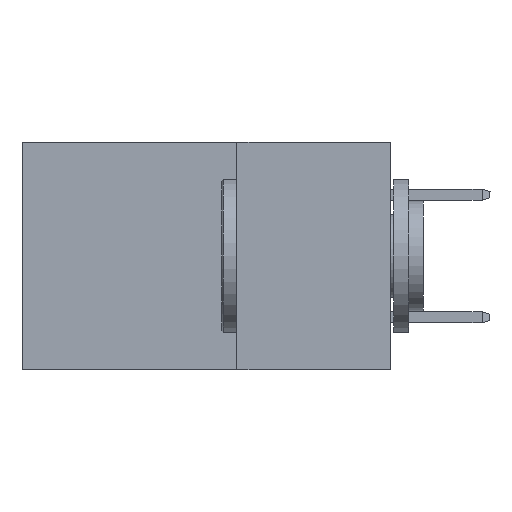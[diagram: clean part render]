
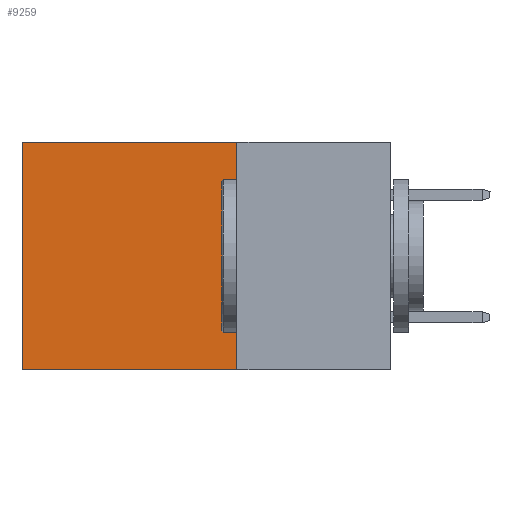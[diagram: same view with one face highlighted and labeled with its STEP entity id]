
A CAD part, left-side view. The second image highlights one B-rep face of the part: STEP entity #9259.
In plain terms, the highlighted planar face has unit normal (-1, 0, 0).
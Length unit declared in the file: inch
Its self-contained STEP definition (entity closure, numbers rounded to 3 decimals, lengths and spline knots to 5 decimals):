
#1408 = LINE ( 'NONE', #2600, #30522 ) ;
#2378 = EDGE_CURVE ( 'NONE', #23301, #19494, #18759, .T. ) ;
#2600 = CARTESIAN_POINT ( 'NONE',  ( 0.2875, 0.6, 0. ) ) ;
#3869 = EDGE_CURVE ( 'NONE', #27335, #26759, #1408, .T. ) ;
#3931 = CARTESIAN_POINT ( 'NONE',  ( 0.2875, 0.25, 0. ) ) ;
#6748 = DIRECTION ( 'NONE',  ( 0., 1., 0. ) ) ;
#7465 = DIRECTION ( 'NONE',  ( 0., 0., -1. ) ) ;
#8483 = CARTESIAN_POINT ( 'NONE',  ( 0.2875, 0.25, -0.37 ) ) ;
#8795 = LINE ( 'NONE', #33313, #10256 ) ;
#9259 = ADVANCED_FACE ( 'NONE', ( #20564 ), #22550, .F. ) ;
#10256 = VECTOR ( 'NONE', #15009, 39.37008 ) ;
#11259 = EDGE_LOOP ( 'NONE', ( #24475, #34367, #26622, #31666 ) ) ;
#12749 = EDGE_CURVE ( 'NONE', #23301, #27335, #38984, .T. ) ;
#13097 = CARTESIAN_POINT ( 'NONE',  ( 0.2875, 0.25, 0. ) ) ;
#13648 = CARTESIAN_POINT ( 'NONE',  ( 0.2875, 0.6, 0. ) ) ;
#15009 = DIRECTION ( 'NONE',  ( 0., 1., 0. ) ) ;
#15402 = AXIS2_PLACEMENT_3D ( 'NONE', #3931, #25070, #34419 ) ;
#18759 = LINE ( 'NONE', #28833, #38855 ) ;
#18828 = CARTESIAN_POINT ( 'NONE',  ( 0.2875, 0.25, 0. ) ) ;
#19494 = VERTEX_POINT ( 'NONE', #8483 ) ;
#20564 = FACE_OUTER_BOUND ( 'NONE', #11259, .T. ) ;
#22550 = PLANE ( 'NONE',  #15402 ) ;
#22758 = VECTOR ( 'NONE', #6748, 39.37008 ) ;
#23301 = VERTEX_POINT ( 'NONE', #18828 ) ;
#24475 = ORIENTED_EDGE ( 'NONE', *, *, #3869, .T. ) ;
#25070 = DIRECTION ( 'NONE',  ( 1., 0., 0. ) ) ;
#26622 = ORIENTED_EDGE ( 'NONE', *, *, #2378, .F. ) ;
#26759 = VERTEX_POINT ( 'NONE', #30993 ) ;
#27335 = VERTEX_POINT ( 'NONE', #13648 ) ;
#28833 = CARTESIAN_POINT ( 'NONE',  ( 0.2875, 0.25, 0. ) ) ;
#30522 = VECTOR ( 'NONE', #7465, 39.37008 ) ;
#30993 = CARTESIAN_POINT ( 'NONE',  ( 0.2875, 0.6, -0.37 ) ) ;
#31666 = ORIENTED_EDGE ( 'NONE', *, *, #12749, .T. ) ;
#31787 = DIRECTION ( 'NONE',  ( 0., 0., -1. ) ) ;
#33313 = CARTESIAN_POINT ( 'NONE',  ( 0.2875, 0.25, -0.37 ) ) ;
#34095 = EDGE_CURVE ( 'NONE', #19494, #26759, #8795, .T. ) ;
#34367 = ORIENTED_EDGE ( 'NONE', *, *, #34095, .F. ) ;
#34419 = DIRECTION ( 'NONE',  ( 0., 0., -1. ) ) ;
#38855 = VECTOR ( 'NONE', #31787, 39.37008 ) ;
#38984 = LINE ( 'NONE', #13097, #22758 ) ;
